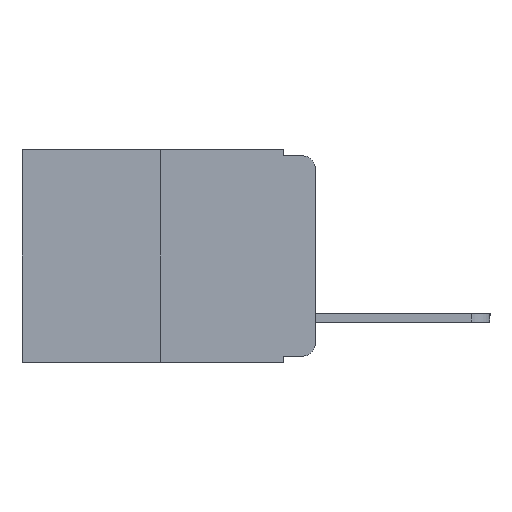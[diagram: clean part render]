
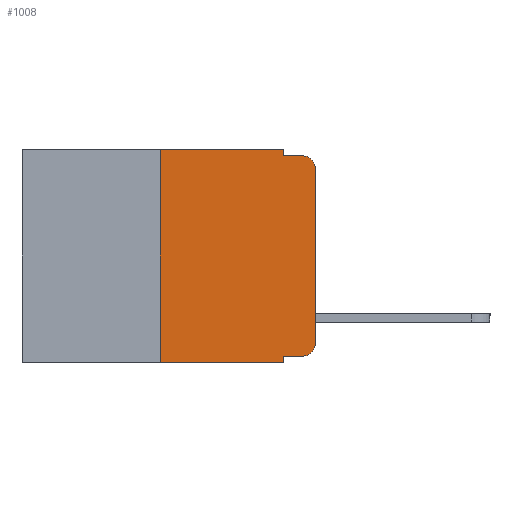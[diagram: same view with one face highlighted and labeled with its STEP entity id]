
A CAD part, left-side view. The second image highlights one B-rep face of the part: STEP entity #1008.
In plain terms, the highlighted planar face has unit normal (-1, 0, 0).
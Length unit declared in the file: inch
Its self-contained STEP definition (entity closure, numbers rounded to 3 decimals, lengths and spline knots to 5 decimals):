
#300 = VERTEX_POINT ( 'NONE', #7933 ) ;
#637 = CARTESIAN_POINT ( 'NONE',  ( 0., 0., -0.313 ) ) ;
#717 = EDGE_CURVE ( 'NONE', #16630, #13498, #21396, .T. ) ;
#1008 = ADVANCED_FACE ( 'NONE', ( #4073 ), #23974, .F. ) ;
#1020 = VECTOR ( 'NONE', #21162, 39.37008 ) ;
#1269 = VECTOR ( 'NONE', #18312, 39.37008 ) ;
#1527 = CARTESIAN_POINT ( 'NONE',  ( 0., 0.473, -0.343 ) ) ;
#1614 = DIRECTION ( 'NONE',  ( 0., -1., 0. ) ) ;
#1885 = VERTEX_POINT ( 'NONE', #20927 ) ;
#2447 = DIRECTION ( 'NONE',  ( -1., 0., 0. ) ) ;
#2808 = LINE ( 'NONE', #16090, #7973 ) ;
#3678 = ORIENTED_EDGE ( 'NONE', *, *, #10139, .T. ) ;
#3723 = LINE ( 'NONE', #5041, #18408 ) ;
#3792 = LINE ( 'NONE', #23029, #24023 ) ;
#4073 = FACE_OUTER_BOUND ( 'NONE', #20457, .T. ) ;
#4540 = CARTESIAN_POINT ( 'NONE',  ( 0., 0.02, -0.01 ) ) ;
#4669 = EDGE_CURVE ( 'NONE', #16630, #1885, #13108, .T. ) ;
#4862 = LINE ( 'NONE', #1527, #14437 ) ;
#5041 = CARTESIAN_POINT ( 'NONE',  ( 0., 0.473, 0. ) ) ;
#5783 = ORIENTED_EDGE ( 'NONE', *, *, #12327, .T. ) ;
#5946 = EDGE_CURVE ( 'NONE', #300, #23088, #2808, .T. ) ;
#6134 = EDGE_CURVE ( 'NONE', #23088, #9918, #3723, .T. ) ;
#6554 = CARTESIAN_POINT ( 'NONE',  ( 0., 0.25, 0. ) ) ;
#6710 = CARTESIAN_POINT ( 'NONE',  ( 0., 0.051, 0. ) ) ;
#6751 = DIRECTION ( 'NONE',  ( 0., -1., 0. ) ) ;
#7010 = ORIENTED_EDGE ( 'NONE', *, *, #8530, .F. ) ;
#7058 = LINE ( 'NONE', #8712, #1269 ) ;
#7933 = CARTESIAN_POINT ( 'NONE',  ( 0., 0.25, -0.343 ) ) ;
#7973 = VECTOR ( 'NONE', #12820, 39.37008 ) ;
#8209 = ORIENTED_EDGE ( 'NONE', *, *, #5946, .F. ) ;
#8530 = EDGE_CURVE ( 'NONE', #9918, #14853, #7058, .T. ) ;
#8712 = CARTESIAN_POINT ( 'NONE',  ( 0., 0.051, 0. ) ) ;
#8906 = DIRECTION ( 'NONE',  ( 0., -1., 0. ) ) ;
#9579 = CARTESIAN_POINT ( 'NONE',  ( 0., 0.051, -0.333 ) ) ;
#9631 = VECTOR ( 'NONE', #6751, 39.37008 ) ;
#9918 = VERTEX_POINT ( 'NONE', #6710 ) ;
#10139 = EDGE_CURVE ( 'NONE', #300, #1885, #4862, .T. ) ;
#11044 = EDGE_CURVE ( 'NONE', #14853, #22819, #20399, .T. ) ;
#11333 = AXIS2_PLACEMENT_3D ( 'NONE', #13953, #2447, #15894 ) ;
#11356 = CARTESIAN_POINT ( 'NONE',  ( 0., 0.02, -0.03 ) ) ;
#11435 = ORIENTED_EDGE ( 'NONE', *, *, #11044, .F. ) ;
#11631 = DIRECTION ( 'NONE',  ( 0., 0., 1. ) ) ;
#12327 = EDGE_CURVE ( 'NONE', #23639, #22819, #20329, .T. ) ;
#12820 = DIRECTION ( 'NONE',  ( 0., 0., 1. ) ) ;
#12830 = CARTESIAN_POINT ( 'NONE',  ( 0., 0.051, -0.01 ) ) ;
#12838 = AXIS2_PLACEMENT_3D ( 'NONE', #22569, #17558, #21140 ) ;
#13108 = LINE ( 'NONE', #23963, #16980 ) ;
#13313 = DIRECTION ( 'NONE',  ( 0., 0., -1. ) ) ;
#13498 = VERTEX_POINT ( 'NONE', #15034 ) ;
#13635 = EDGE_CURVE ( 'NONE', #15865, #23639, #3792, .T. ) ;
#13880 = ORIENTED_EDGE ( 'NONE', *, *, #4669, .F. ) ;
#13953 = CARTESIAN_POINT ( 'NONE',  ( 0., 0.02, -0.313 ) ) ;
#14437 = VECTOR ( 'NONE', #1614, 39.37008 ) ;
#14771 = ORIENTED_EDGE ( 'NONE', *, *, #13635, .T. ) ;
#14853 = VERTEX_POINT ( 'NONE', #12830 ) ;
#15034 = CARTESIAN_POINT ( 'NONE',  ( 0., 0.02, -0.333 ) ) ;
#15337 = DIRECTION ( 'NONE',  ( 0., 0., -1. ) ) ;
#15865 = VERTEX_POINT ( 'NONE', #637 ) ;
#15894 = DIRECTION ( 'NONE',  ( 0., 0., -1. ) ) ;
#16090 = CARTESIAN_POINT ( 'NONE',  ( 0., 0.25, 0. ) ) ;
#16226 = CIRCLE ( 'NONE', #11333, 0.02 ) ;
#16630 = VERTEX_POINT ( 'NONE', #9579 ) ;
#16980 = VECTOR ( 'NONE', #15337, 39.37008 ) ;
#17558 = DIRECTION ( 'NONE',  ( 1., 0., 0. ) ) ;
#17735 = AXIS2_PLACEMENT_3D ( 'NONE', #11356, #24617, #13313 ) ;
#18312 = DIRECTION ( 'NONE',  ( 0., 0., -1. ) ) ;
#18408 = VECTOR ( 'NONE', #8906, 39.37008 ) ;
#18975 = ORIENTED_EDGE ( 'NONE', *, *, #717, .T. ) ;
#19426 = CARTESIAN_POINT ( 'NONE',  ( 0., 0.051, -0.333 ) ) ;
#20129 = CARTESIAN_POINT ( 'NONE',  ( 0., 0.051, -0.01 ) ) ;
#20329 = CIRCLE ( 'NONE', #17735, 0.02 ) ;
#20399 = LINE ( 'NONE', #20129, #9631 ) ;
#20457 = EDGE_LOOP ( 'NONE', ( #14771, #5783, #11435, #7010, #22759, #8209, #3678, #13880, #18975, #24496 ) ) ;
#20927 = CARTESIAN_POINT ( 'NONE',  ( 0., 0.051, -0.343 ) ) ;
#21140 = DIRECTION ( 'NONE',  ( 0., 0., -1. ) ) ;
#21162 = DIRECTION ( 'NONE',  ( 0., -1., 0. ) ) ;
#21396 = LINE ( 'NONE', #19426, #1020 ) ;
#21515 = CARTESIAN_POINT ( 'NONE',  ( 0., 0., -0.03 ) ) ;
#22569 = CARTESIAN_POINT ( 'NONE',  ( 0., 0.473, 0. ) ) ;
#22759 = ORIENTED_EDGE ( 'NONE', *, *, #6134, .F. ) ;
#22819 = VERTEX_POINT ( 'NONE', #4540 ) ;
#23029 = CARTESIAN_POINT ( 'NONE',  ( 0., 0., 0. ) ) ;
#23088 = VERTEX_POINT ( 'NONE', #6554 ) ;
#23639 = VERTEX_POINT ( 'NONE', #21515 ) ;
#23963 = CARTESIAN_POINT ( 'NONE',  ( 0., 0.051, 0. ) ) ;
#23974 = PLANE ( 'NONE',  #12838 ) ;
#24023 = VECTOR ( 'NONE', #11631, 39.37008 ) ;
#24236 = EDGE_CURVE ( 'NONE', #13498, #15865, #16226, .T. ) ;
#24496 = ORIENTED_EDGE ( 'NONE', *, *, #24236, .T. ) ;
#24617 = DIRECTION ( 'NONE',  ( -1., 0., 0. ) ) ;
